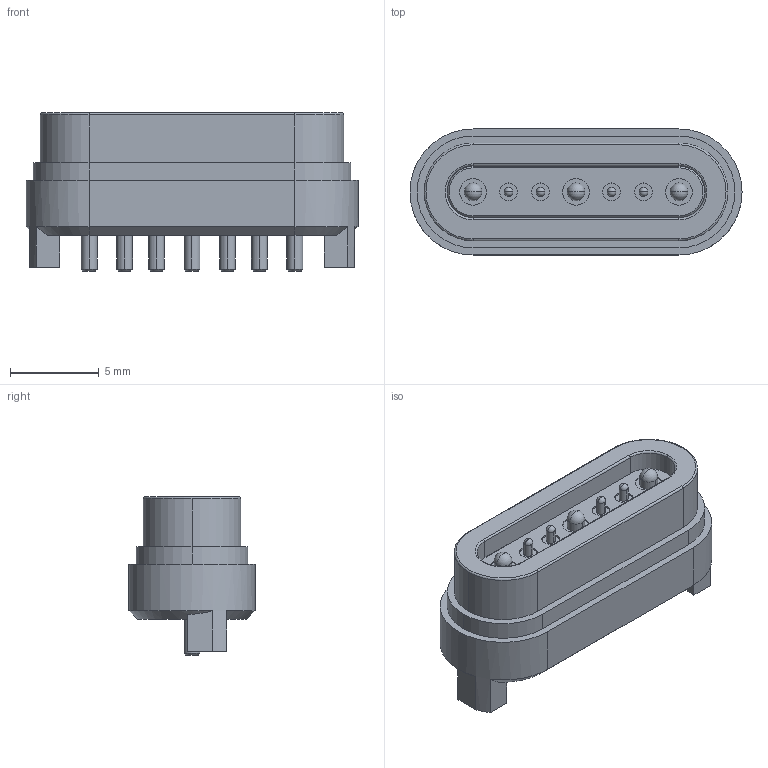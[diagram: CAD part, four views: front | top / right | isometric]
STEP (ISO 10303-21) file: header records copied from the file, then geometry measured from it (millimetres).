
FILE_DESCRIPTION (( 'STEP AP203' ), '1' );
FILE_NAME ('685-C0722210115.STEP', '2023-02-15T10:03:57', ( 'Magnum' ), ( '' ), 'SwSTEP 2.0', 'SolidWorks 2020', '' );
FILE_SCHEMA (( 'CONFIG_CONTROL_DESIGN' ));
Length unit declared in the file: millimetre
Products named in the file (1): 685-C0722210115
Bounding box: 18.7 x 7.1 x 8.9 mm (x, y, z)
Volume: 692.6 mm3; surface area: 955.9 mm2
Topology: 1 solids, 10 shells, 210 faces, 475 edges, 296 vertices
Faces by surface type: cylinder 91, plane 78, cone 21, sphere 14, torus 6
Entity records: 5935 total; most frequent: DIRECTION 1112, CARTESIAN_POINT 1002, ORIENTED_EDGE 922, EDGE_CURVE 461, AXIS2_PLACEMENT_3D 448, VERTEX_POINT 296, EDGE_LOOP 249, CIRCLE 237
